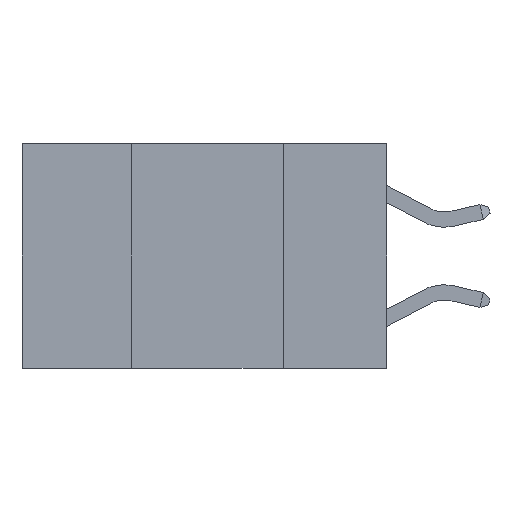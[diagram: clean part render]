
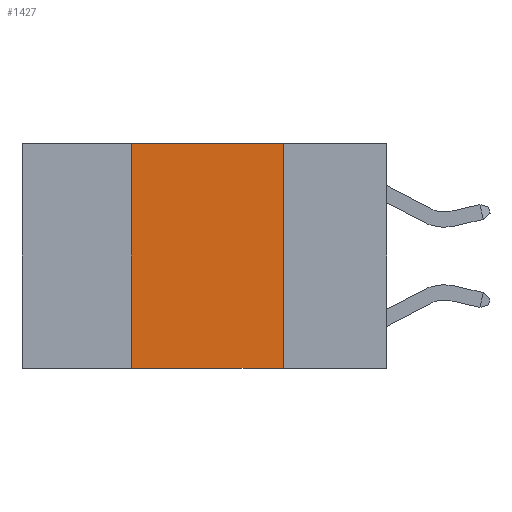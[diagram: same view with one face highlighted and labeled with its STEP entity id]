
A CAD part, left-side view. The second image highlights one B-rep face of the part: STEP entity #1427.
In plain terms, the highlighted planar face has unit normal (-1, 0, 0).
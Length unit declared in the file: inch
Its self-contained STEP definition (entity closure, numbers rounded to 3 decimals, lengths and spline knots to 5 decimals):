
#9 = CARTESIAN_POINT ( 'NONE',  ( 0., 0.6, 0. ) ) ;
#60 = ORIENTED_EDGE ( 'NONE', *, *, #971, .F. ) ;
#537 = LINE ( 'NONE', #3372, #6064 ) ;
#811 = DIRECTION ( 'NONE',  ( 0., 0., -1. ) ) ;
#896 = CARTESIAN_POINT ( 'NONE',  ( 0., 0.17, -0.37 ) ) ;
#971 = EDGE_CURVE ( 'NONE', #4265, #7550, #537, .T. ) ;
#1007 = DIRECTION ( 'NONE',  ( 0., -1., 0. ) ) ;
#1346 = LINE ( 'NONE', #8931, #1677 ) ;
#1427 = ADVANCED_FACE ( 'NONE', ( #12076 ), #7896, .F. ) ;
#1677 = VECTOR ( 'NONE', #3960, 39.37008 ) ;
#3372 = CARTESIAN_POINT ( 'NONE',  ( 0., 0.17, 0. ) ) ;
#3960 = DIRECTION ( 'NONE',  ( 0., 0., 1. ) ) ;
#4070 = EDGE_LOOP ( 'NONE', ( #60, #5624, #5936, #8562 ) ) ;
#4265 = VERTEX_POINT ( 'NONE', #12072 ) ;
#4423 = VECTOR ( 'NONE', #9192, 39.37008 ) ;
#5531 = CARTESIAN_POINT ( 'NONE',  ( 0., 0.42, -0.37 ) ) ;
#5624 = ORIENTED_EDGE ( 'NONE', *, *, #6416, .F. ) ;
#5936 = ORIENTED_EDGE ( 'NONE', *, *, #6915, .F. ) ;
#6064 = VECTOR ( 'NONE', #10261, 39.37008 ) ;
#6416 = EDGE_CURVE ( 'NONE', #9399, #4265, #7108, .T. ) ;
#6915 = EDGE_CURVE ( 'NONE', #9777, #9399, #1346, .T. ) ;
#6932 = DIRECTION ( 'NONE',  ( 1., 0., 0. ) ) ;
#7108 = LINE ( 'NONE', #9, #4423 ) ;
#7550 = VERTEX_POINT ( 'NONE', #896 ) ;
#7896 = PLANE ( 'NONE',  #9899 ) ;
#8056 = CARTESIAN_POINT ( 'NONE',  ( 0., 0.42, 0. ) ) ;
#8134 = CARTESIAN_POINT ( 'NONE',  ( 0., 0.6, -0.37 ) ) ;
#8562 = ORIENTED_EDGE ( 'NONE', *, *, #8811, .T. ) ;
#8596 = VECTOR ( 'NONE', #1007, 39.37008 ) ;
#8811 = EDGE_CURVE ( 'NONE', #9777, #7550, #9474, .T. ) ;
#8931 = CARTESIAN_POINT ( 'NONE',  ( 0., 0.42, 0. ) ) ;
#9192 = DIRECTION ( 'NONE',  ( 0., -1., 0. ) ) ;
#9399 = VERTEX_POINT ( 'NONE', #8056 ) ;
#9474 = LINE ( 'NONE', #8134, #8596 ) ;
#9777 = VERTEX_POINT ( 'NONE', #5531 ) ;
#9899 = AXIS2_PLACEMENT_3D ( 'NONE', #10794, #6932, #811 ) ;
#10261 = DIRECTION ( 'NONE',  ( 0., 0., -1. ) ) ;
#10794 = CARTESIAN_POINT ( 'NONE',  ( 0., 0.6, 0. ) ) ;
#12072 = CARTESIAN_POINT ( 'NONE',  ( 0., 0.17, 0. ) ) ;
#12076 = FACE_OUTER_BOUND ( 'NONE', #4070, .T. ) ;
